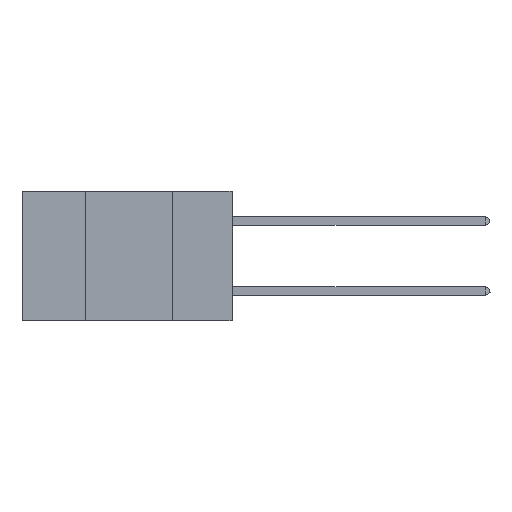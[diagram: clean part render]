
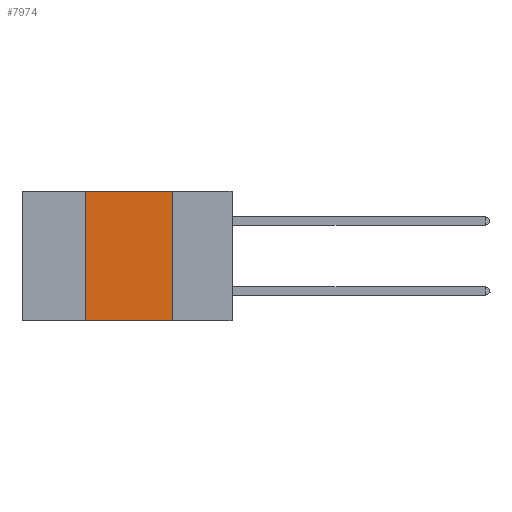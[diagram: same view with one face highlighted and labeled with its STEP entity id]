
A CAD part, left-side view. The second image highlights one B-rep face of the part: STEP entity #7974.
In plain terms, the highlighted planar face has unit normal (-1, 0, 0).
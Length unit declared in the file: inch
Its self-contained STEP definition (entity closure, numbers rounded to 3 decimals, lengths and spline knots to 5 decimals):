
#207 = VECTOR ( 'NONE', #8004, 39.37008 ) ;
#282 = VECTOR ( 'NONE', #6060, 39.37008 ) ;
#1770 = EDGE_CURVE ( 'NONE', #2616, #9078, #8351, .T. ) ;
#2009 = LINE ( 'NONE', #7543, #4297 ) ;
#2616 = VERTEX_POINT ( 'NONE', #10127 ) ;
#4072 = DIRECTION ( 'NONE',  ( 0., -1., 0. ) ) ;
#4297 = VECTOR ( 'NONE', #10577, 39.37008 ) ;
#4490 = EDGE_CURVE ( 'NONE', #2616, #8269, #7923, .T. ) ;
#4570 = CARTESIAN_POINT ( 'NONE',  ( 0., 0.42, 0. ) ) ;
#4862 = ORIENTED_EDGE ( 'NONE', *, *, #5351, .F. ) ;
#5351 = EDGE_CURVE ( 'NONE', #12843, #8269, #2009, .T. ) ;
#6060 = DIRECTION ( 'NONE',  ( 0., -1., 0. ) ) ;
#6959 = PLANE ( 'NONE',  #7077 ) ;
#7077 = AXIS2_PLACEMENT_3D ( 'NONE', #10077, #12076, #8069 ) ;
#7543 = CARTESIAN_POINT ( 'NONE',  ( 0., 0.17, 0. ) ) ;
#7566 = ORIENTED_EDGE ( 'NONE', *, *, #7657, .F. ) ;
#7657 = EDGE_CURVE ( 'NONE', #9078, #12843, #10384, .T. ) ;
#7902 = EDGE_LOOP ( 'NONE', ( #4862, #7566, #10833, #13267 ) ) ;
#7923 = LINE ( 'NONE', #12193, #282 ) ;
#7974 = ADVANCED_FACE ( 'NONE', ( #10704 ), #6959, .F. ) ;
#8004 = DIRECTION ( 'NONE',  ( 0., 0., 1. ) ) ;
#8069 = DIRECTION ( 'NONE',  ( 0., 0., -1. ) ) ;
#8269 = VERTEX_POINT ( 'NONE', #9717 ) ;
#8351 = LINE ( 'NONE', #9753, #207 ) ;
#9078 = VERTEX_POINT ( 'NONE', #4570 ) ;
#9717 = CARTESIAN_POINT ( 'NONE',  ( 0., 0.17, -0.37 ) ) ;
#9753 = CARTESIAN_POINT ( 'NONE',  ( 0., 0.42, 0. ) ) ;
#10045 = VECTOR ( 'NONE', #4072, 39.37008 ) ;
#10077 = CARTESIAN_POINT ( 'NONE',  ( 0., 0.6, 0. ) ) ;
#10127 = CARTESIAN_POINT ( 'NONE',  ( 0., 0.42, -0.37 ) ) ;
#10305 = CARTESIAN_POINT ( 'NONE',  ( 0., 0.6, 0. ) ) ;
#10384 = LINE ( 'NONE', #10305, #10045 ) ;
#10577 = DIRECTION ( 'NONE',  ( 0., 0., -1. ) ) ;
#10704 = FACE_OUTER_BOUND ( 'NONE', #7902, .T. ) ;
#10833 = ORIENTED_EDGE ( 'NONE', *, *, #1770, .F. ) ;
#11057 = CARTESIAN_POINT ( 'NONE',  ( 0., 0.17, 0. ) ) ;
#12076 = DIRECTION ( 'NONE',  ( 1., 0., 0. ) ) ;
#12193 = CARTESIAN_POINT ( 'NONE',  ( 0., 0.6, -0.37 ) ) ;
#12843 = VERTEX_POINT ( 'NONE', #11057 ) ;
#13267 = ORIENTED_EDGE ( 'NONE', *, *, #4490, .T. ) ;
